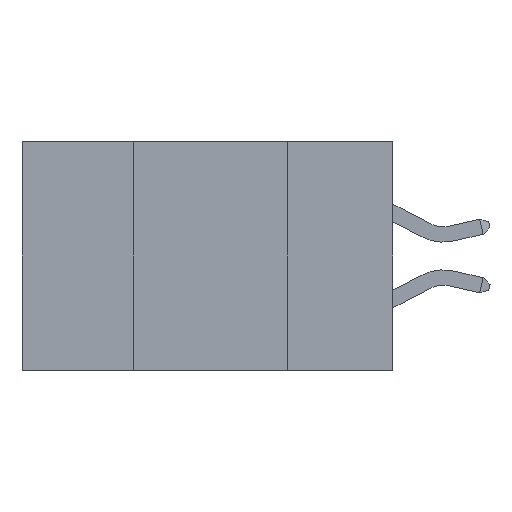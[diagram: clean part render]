
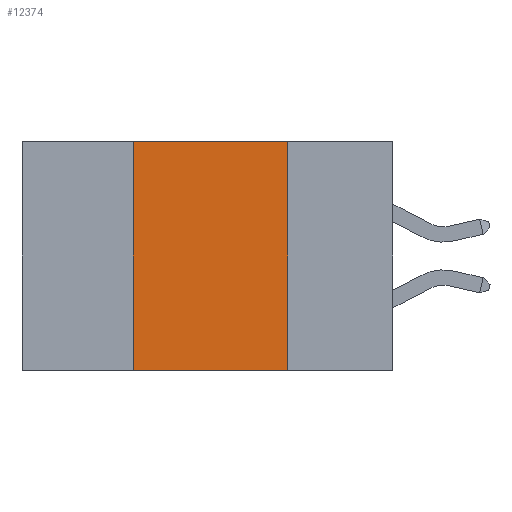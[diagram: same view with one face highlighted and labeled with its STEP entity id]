
A CAD part, left-side view. The second image highlights one B-rep face of the part: STEP entity #12374.
In plain terms, the highlighted planar face has unit normal (-1, 0, 0).
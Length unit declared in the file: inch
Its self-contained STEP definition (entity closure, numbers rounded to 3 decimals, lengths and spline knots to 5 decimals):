
#133 = CARTESIAN_POINT ( 'NONE',  ( 0., 0.42, -0.37 ) ) ;
#534 = LINE ( 'NONE', #12366, #13601 ) ;
#904 = CARTESIAN_POINT ( 'NONE',  ( 0., 0.17, 0. ) ) ;
#1503 = VECTOR ( 'NONE', #11166, 39.37008 ) ;
#3625 = VERTEX_POINT ( 'NONE', #20837 ) ;
#4839 = EDGE_CURVE ( 'NONE', #27616, #6907, #12001, .T. ) ;
#5297 = DIRECTION ( 'NONE',  ( 1., 0., 0. ) ) ;
#6907 = VERTEX_POINT ( 'NONE', #904 ) ;
#7189 = ORIENTED_EDGE ( 'NONE', *, *, #24935, .T. ) ;
#10529 = CARTESIAN_POINT ( 'NONE',  ( 0., 0.6, 0. ) ) ;
#11166 = DIRECTION ( 'NONE',  ( 0., 0., 1. ) ) ;
#12001 = LINE ( 'NONE', #27503, #12906 ) ;
#12366 = CARTESIAN_POINT ( 'NONE',  ( 0., 0.6, -0.37 ) ) ;
#12374 = ADVANCED_FACE ( 'NONE', ( #26882 ), #29264, .F. ) ;
#12651 = AXIS2_PLACEMENT_3D ( 'NONE', #10529, #5297, #30310 ) ;
#12906 = VECTOR ( 'NONE', #24616, 39.37008 ) ;
#13601 = VECTOR ( 'NONE', #34343, 39.37008 ) ;
#13699 = ORIENTED_EDGE ( 'NONE', *, *, #28083, .F. ) ;
#14533 = LINE ( 'NONE', #35820, #1503 ) ;
#18838 = CARTESIAN_POINT ( 'NONE',  ( 0., 0.17, 0. ) ) ;
#19313 = ORIENTED_EDGE ( 'NONE', *, *, #4839, .F. ) ;
#20837 = CARTESIAN_POINT ( 'NONE',  ( 0., 0.17, -0.37 ) ) ;
#21857 = DIRECTION ( 'NONE',  ( 0., 0., -1. ) ) ;
#23765 = CARTESIAN_POINT ( 'NONE',  ( 0., 0.42, 0. ) ) ;
#23805 = ORIENTED_EDGE ( 'NONE', *, *, #34527, .F. ) ;
#23969 = LINE ( 'NONE', #18838, #24372 ) ;
#24372 = VECTOR ( 'NONE', #21857, 39.37008 ) ;
#24616 = DIRECTION ( 'NONE',  ( 0., -1., 0. ) ) ;
#24935 = EDGE_CURVE ( 'NONE', #35225, #3625, #534, .T. ) ;
#26882 = FACE_OUTER_BOUND ( 'NONE', #28587, .T. ) ;
#27503 = CARTESIAN_POINT ( 'NONE',  ( 0., 0.6, 0. ) ) ;
#27616 = VERTEX_POINT ( 'NONE', #23765 ) ;
#28083 = EDGE_CURVE ( 'NONE', #35225, #27616, #14533, .T. ) ;
#28587 = EDGE_LOOP ( 'NONE', ( #23805, #19313, #13699, #7189 ) ) ;
#29264 = PLANE ( 'NONE',  #12651 ) ;
#30310 = DIRECTION ( 'NONE',  ( 0., 0., -1. ) ) ;
#34343 = DIRECTION ( 'NONE',  ( 0., -1., 0. ) ) ;
#34527 = EDGE_CURVE ( 'NONE', #6907, #3625, #23969, .T. ) ;
#35225 = VERTEX_POINT ( 'NONE', #133 ) ;
#35820 = CARTESIAN_POINT ( 'NONE',  ( 0., 0.42, 0. ) ) ;
